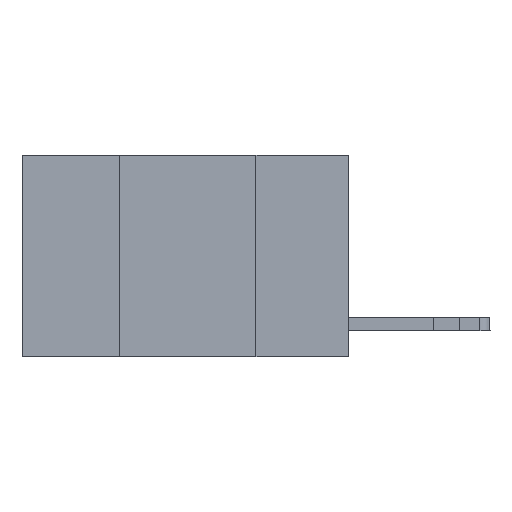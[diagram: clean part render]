
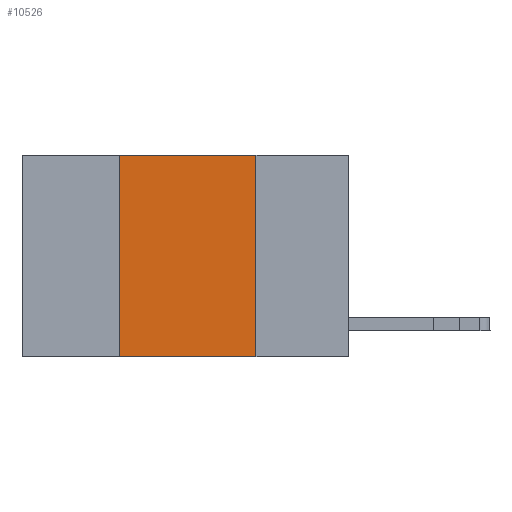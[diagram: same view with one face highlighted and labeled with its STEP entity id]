
A CAD part, left-side view. The second image highlights one B-rep face of the part: STEP entity #10526.
In plain terms, the highlighted planar face has unit normal (-1, 0, 0).
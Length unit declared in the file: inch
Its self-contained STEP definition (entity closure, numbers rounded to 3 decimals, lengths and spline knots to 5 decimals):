
#139 = ORIENTED_EDGE ( 'NONE', *, *, #8700, .F. ) ;
#203 = DIRECTION ( 'NONE',  ( 0., -1., 0. ) ) ;
#290 = CARTESIAN_POINT ( 'NONE',  ( 0., 0.42, 0. ) ) ;
#488 = LINE ( 'NONE', #1111, #9821 ) ;
#972 = ORIENTED_EDGE ( 'NONE', *, *, #8119, .T. ) ;
#1111 = CARTESIAN_POINT ( 'NONE',  ( 0., 0.17, 0. ) ) ;
#1273 = DIRECTION ( 'NONE',  ( 0., 0., -1. ) ) ;
#2139 = EDGE_CURVE ( 'NONE', #10596, #6344, #2575, .T. ) ;
#2575 = LINE ( 'NONE', #5499, #7346 ) ;
#2849 = ORIENTED_EDGE ( 'NONE', *, *, #3051, .F. ) ;
#2888 = DIRECTION ( 'NONE',  ( 0., 0., 1. ) ) ;
#3020 = DIRECTION ( 'NONE',  ( 1., 0., 0. ) ) ;
#3051 = EDGE_CURVE ( 'NONE', #5505, #10596, #5517, .T. ) ;
#4740 = PLANE ( 'NONE',  #10329 ) ;
#5499 = CARTESIAN_POINT ( 'NONE',  ( 0., 0.6, 0. ) ) ;
#5505 = VERTEX_POINT ( 'NONE', #7207 ) ;
#5517 = LINE ( 'NONE', #9082, #7993 ) ;
#5581 = CARTESIAN_POINT ( 'NONE',  ( 0., 0.6, 0. ) ) ;
#5705 = FACE_OUTER_BOUND ( 'NONE', #11159, .T. ) ;
#5957 = VERTEX_POINT ( 'NONE', #6461 ) ;
#6344 = VERTEX_POINT ( 'NONE', #8155 ) ;
#6461 = CARTESIAN_POINT ( 'NONE',  ( 0., 0.17, -0.37 ) ) ;
#7207 = CARTESIAN_POINT ( 'NONE',  ( 0., 0.42, -0.37 ) ) ;
#7346 = VECTOR ( 'NONE', #8159, 39.37008 ) ;
#7743 = VECTOR ( 'NONE', #203, 39.37008 ) ;
#7993 = VECTOR ( 'NONE', #2888, 39.37008 ) ;
#8119 = EDGE_CURVE ( 'NONE', #5505, #5957, #9062, .T. ) ;
#8155 = CARTESIAN_POINT ( 'NONE',  ( 0., 0.17, 0. ) ) ;
#8159 = DIRECTION ( 'NONE',  ( 0., -1., 0. ) ) ;
#8349 = DIRECTION ( 'NONE',  ( 0., 0., -1. ) ) ;
#8700 = EDGE_CURVE ( 'NONE', #6344, #5957, #488, .T. ) ;
#9062 = LINE ( 'NONE', #9116, #7743 ) ;
#9082 = CARTESIAN_POINT ( 'NONE',  ( 0., 0.42, 0. ) ) ;
#9116 = CARTESIAN_POINT ( 'NONE',  ( 0., 0.6, -0.37 ) ) ;
#9821 = VECTOR ( 'NONE', #1273, 39.37008 ) ;
#10329 = AXIS2_PLACEMENT_3D ( 'NONE', #5581, #3020, #8349 ) ;
#10526 = ADVANCED_FACE ( 'NONE', ( #5705 ), #4740, .F. ) ;
#10596 = VERTEX_POINT ( 'NONE', #290 ) ;
#11017 = ORIENTED_EDGE ( 'NONE', *, *, #2139, .F. ) ;
#11159 = EDGE_LOOP ( 'NONE', ( #139, #11017, #2849, #972 ) ) ;
